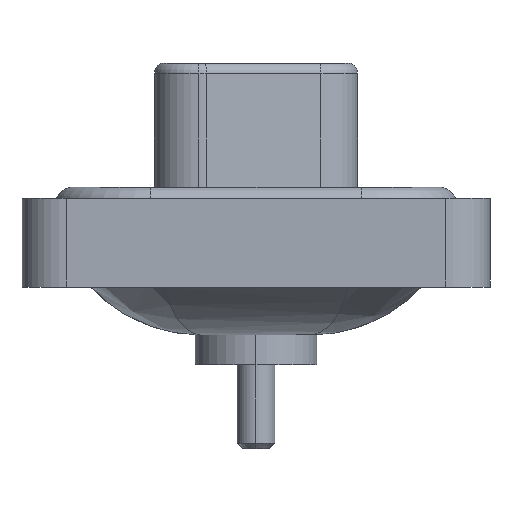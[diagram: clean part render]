
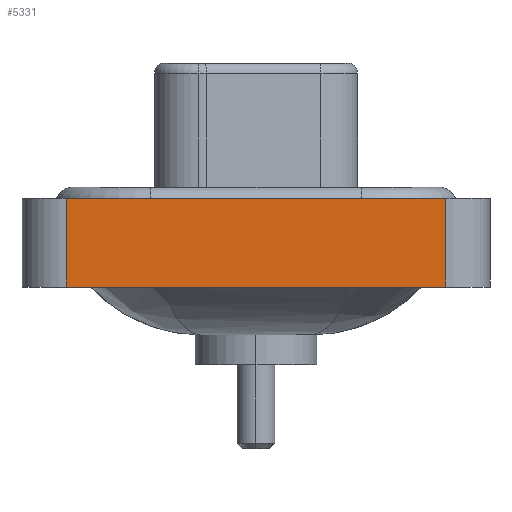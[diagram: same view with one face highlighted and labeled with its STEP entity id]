
A CAD part, left-side view. The second image highlights one B-rep face of the part: STEP entity #5331.
In plain terms, the highlighted planar face has unit normal (-1, 0, 0).
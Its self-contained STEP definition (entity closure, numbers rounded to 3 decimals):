
#130 = CARTESIAN_POINT ( 'NONE',  ( -7.25, -8.55, -3.6 ) ) ;
#195 = ORIENTED_EDGE ( 'NONE', *, *, #3817, .T. ) ;
#892 = CARTESIAN_POINT ( 'NONE',  ( -7.25, -8.55, -3.6 ) ) ;
#914 = CARTESIAN_POINT ( 'NONE',  ( -7.25, 8.55, -3.6 ) ) ;
#1003 = EDGE_CURVE ( 'NONE', #7181, #7626, #9155, .T. ) ;
#2269 = VECTOR ( 'NONE', #4298, 1000. ) ;
#2479 = AXIS2_PLACEMENT_3D ( 'NONE', #2777, #5565, #2588 ) ;
#2588 = DIRECTION ( 'NONE',  ( 0., 0., 1. ) ) ;
#2777 = CARTESIAN_POINT ( 'NONE',  ( -7.25, -8.55, -3.6 ) ) ;
#3170 = DIRECTION ( 'NONE',  ( 0., 0., 1. ) ) ;
#3547 = EDGE_CURVE ( 'NONE', #7626, #7420, #9699, .T. ) ;
#3817 = EDGE_CURVE ( 'NONE', #7181, #12211, #13789, .T. ) ;
#3938 = CARTESIAN_POINT ( 'NONE',  ( -7.25, 8.55, 0.4 ) ) ;
#3968 = ORIENTED_EDGE ( 'NONE', *, *, #7491, .T. ) ;
#4298 = DIRECTION ( 'NONE',  ( 0., -1., 0. ) ) ;
#5331 = ADVANCED_FACE ( 'NONE', ( #9587 ), #6628, .T. ) ;
#5460 = EDGE_LOOP ( 'NONE', ( #3968, #12384, #7107, #195 ) ) ;
#5565 = DIRECTION ( 'NONE',  ( -1., 0., 0. ) ) ;
#5632 = CARTESIAN_POINT ( 'NONE',  ( -7.25, -8.55, -3.6 ) ) ;
#6628 = PLANE ( 'NONE',  #2479 ) ;
#6726 = VECTOR ( 'NONE', #14543, 1000. ) ;
#7107 = ORIENTED_EDGE ( 'NONE', *, *, #1003, .F. ) ;
#7181 = VERTEX_POINT ( 'NONE', #15715 ) ;
#7420 = VERTEX_POINT ( 'NONE', #8089 ) ;
#7491 = EDGE_CURVE ( 'NONE', #12211, #7420, #14035, .T. ) ;
#7626 = VERTEX_POINT ( 'NONE', #3938 ) ;
#8089 = CARTESIAN_POINT ( 'NONE',  ( -7.25, -8.55, 0.4 ) ) ;
#8353 = DIRECTION ( 'NONE',  ( 0., -1., 0. ) ) ;
#8482 = VECTOR ( 'NONE', #8353, 1000. ) ;
#8539 = CARTESIAN_POINT ( 'NONE',  ( -7.25, -8.55, 0.4 ) ) ;
#9155 = LINE ( 'NONE', #914, #6726 ) ;
#9587 = FACE_OUTER_BOUND ( 'NONE', #5460, .T. ) ;
#9699 = LINE ( 'NONE', #8539, #8482 ) ;
#12211 = VERTEX_POINT ( 'NONE', #892 ) ;
#12384 = ORIENTED_EDGE ( 'NONE', *, *, #3547, .F. ) ;
#13789 = LINE ( 'NONE', #5632, #2269 ) ;
#14035 = LINE ( 'NONE', #130, #17032 ) ;
#14543 = DIRECTION ( 'NONE',  ( 0., 0., 1. ) ) ;
#15715 = CARTESIAN_POINT ( 'NONE',  ( -7.25, 8.55, -3.6 ) ) ;
#17032 = VECTOR ( 'NONE', #3170, 1000. ) ;
